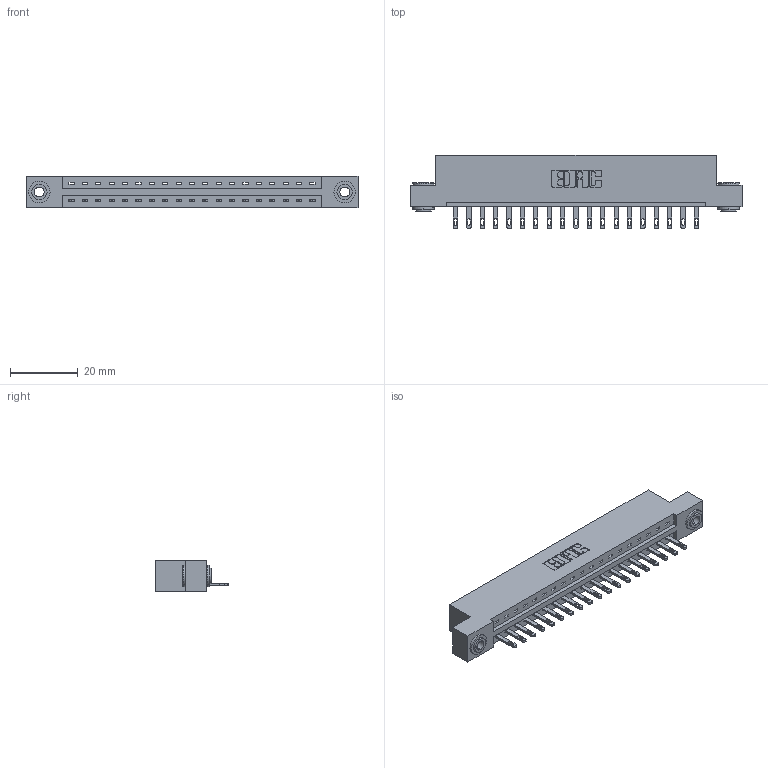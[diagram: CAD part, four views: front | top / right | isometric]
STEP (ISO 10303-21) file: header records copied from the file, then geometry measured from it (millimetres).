
FILE_DESCRIPTION (( 'STEP AP203' ), '1' );
FILE_NAME ('887-019-500-103.STEP', '2020-09-20T17:53:24', ( '' ), ( '' ), 'SwSTEP 2.0', 'SolidWorks 2020', '' );
FILE_SCHEMA (( 'CONFIG_CONTROL_DESIGN' ));
Length unit declared in the file: inch
Products named in the file (4): 887-019-500-103; 837 Part_Flush Mounting Lugs - 0.156 Dia-TH; 345-250-002_345-250-002-102; 345-292-001_345-293-100
Assembly tree (22 placements, depth 2):
  887-019-500-103
    837 Part_Flush Mounting Lugs - 0.156 Dia-TH
    345-292-001_345-293-100  x19
    345-250-002_345-250-002-102  x2
Bounding box: 98.3 x 21.85 x 9.4 mm (x, y, z)
Volume: 9959.8 mm3; surface area: 10441.4 mm2
Topology: 22 solids, 22 shells, 1254 faces, 3807 edges, 2534 vertices
Faces by surface type: plane 840, cylinder 406, cone 8
Entity records: 17678 total; most frequent: CARTESIAN_POINT 3054, ORIENTED_EDGE 3002, DIRECTION 2653, EDGE_CURVE 1501, LINE 1345, VECTOR 1345, VERTEX_POINT 998, AXIS2_PLACEMENT_3D 654
